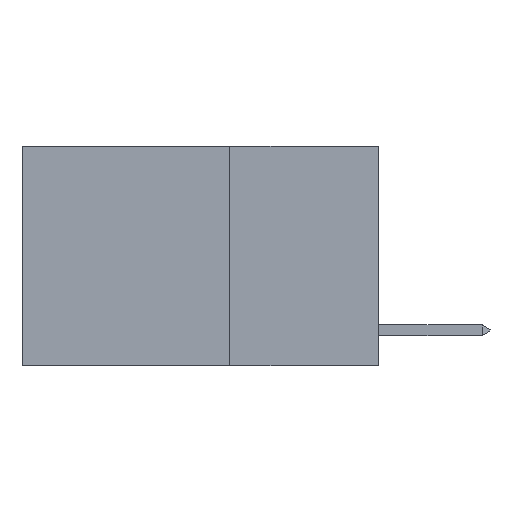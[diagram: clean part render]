
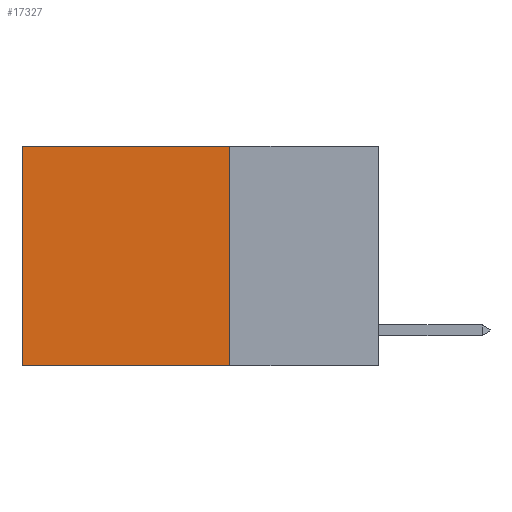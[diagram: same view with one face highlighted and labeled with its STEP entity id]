
A CAD part, left-side view. The second image highlights one B-rep face of the part: STEP entity #17327.
In plain terms, the highlighted planar face has unit normal (-1, 0, 0).
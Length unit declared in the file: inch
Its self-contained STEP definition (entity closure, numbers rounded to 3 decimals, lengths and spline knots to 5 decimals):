
#125 = CARTESIAN_POINT ( 'NONE',  ( 0.2625, 0.25, -0.37 ) ) ;
#239 = ORIENTED_EDGE ( 'NONE', *, *, #13217, .T. ) ;
#435 = VECTOR ( 'NONE', #7815, 39.37008 ) ;
#680 = CARTESIAN_POINT ( 'NONE',  ( 0.2625, 0.25, -0.37 ) ) ;
#1504 = EDGE_CURVE ( 'NONE', #14923, #2404, #15375, .T. ) ;
#2106 = EDGE_CURVE ( 'NONE', #19870, #14923, #12575, .T. ) ;
#2404 = VERTEX_POINT ( 'NONE', #8750 ) ;
#3731 = DIRECTION ( 'NONE',  ( 0., 1., 0. ) ) ;
#4237 = LINE ( 'NONE', #15480, #15418 ) ;
#5046 = CARTESIAN_POINT ( 'NONE',  ( 0.2625, 0.6, 0. ) ) ;
#6069 = EDGE_CURVE ( 'NONE', #19870, #10499, #8008, .T. ) ;
#6143 = CARTESIAN_POINT ( 'NONE',  ( 0.2625, 0.25, 0. ) ) ;
#6171 = EDGE_LOOP ( 'NONE', ( #239, #8170, #20754, #18900 ) ) ;
#6232 = DIRECTION ( 'NONE',  ( 0., 0., -1. ) ) ;
#6233 = DIRECTION ( 'NONE',  ( 0., 1., 0. ) ) ;
#6431 = VECTOR ( 'NONE', #6233, 39.37008 ) ;
#7492 = DIRECTION ( 'NONE',  ( 0., 0., -1. ) ) ;
#7712 = PLANE ( 'NONE',  #17352 ) ;
#7815 = DIRECTION ( 'NONE',  ( 0., 0., -1. ) ) ;
#8008 = LINE ( 'NONE', #17478, #6431 ) ;
#8170 = ORIENTED_EDGE ( 'NONE', *, *, #1504, .F. ) ;
#8750 = CARTESIAN_POINT ( 'NONE',  ( 0.2625, 0.6, -0.37 ) ) ;
#10499 = VERTEX_POINT ( 'NONE', #5046 ) ;
#12575 = LINE ( 'NONE', #20254, #435 ) ;
#13217 = EDGE_CURVE ( 'NONE', #10499, #2404, #4237, .T. ) ;
#14652 = CARTESIAN_POINT ( 'NONE',  ( 0.2625, 0.25, 0. ) ) ;
#14832 = VECTOR ( 'NONE', #3731, 39.37008 ) ;
#14923 = VERTEX_POINT ( 'NONE', #125 ) ;
#15375 = LINE ( 'NONE', #680, #14832 ) ;
#15418 = VECTOR ( 'NONE', #7492, 39.37008 ) ;
#15480 = CARTESIAN_POINT ( 'NONE',  ( 0.2625, 0.6, 0. ) ) ;
#17270 = FACE_OUTER_BOUND ( 'NONE', #6171, .T. ) ;
#17327 = ADVANCED_FACE ( 'NONE', ( #17270 ), #7712, .F. ) ;
#17352 = AXIS2_PLACEMENT_3D ( 'NONE', #6143, #20650, #6232 ) ;
#17478 = CARTESIAN_POINT ( 'NONE',  ( 0.2625, 0.25, 0. ) ) ;
#18900 = ORIENTED_EDGE ( 'NONE', *, *, #6069, .T. ) ;
#19870 = VERTEX_POINT ( 'NONE', #14652 ) ;
#20254 = CARTESIAN_POINT ( 'NONE',  ( 0.2625, 0.25, 0. ) ) ;
#20650 = DIRECTION ( 'NONE',  ( 1., 0., 0. ) ) ;
#20754 = ORIENTED_EDGE ( 'NONE', *, *, #2106, .F. ) ;
